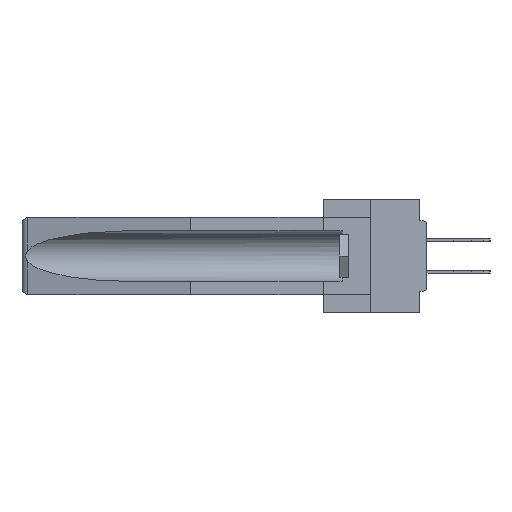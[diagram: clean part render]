
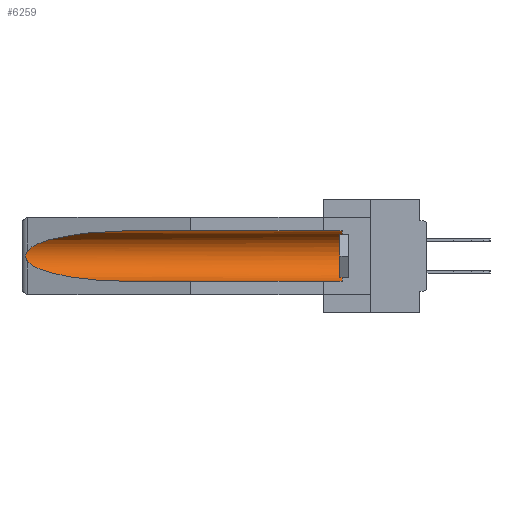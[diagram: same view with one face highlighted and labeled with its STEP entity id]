
A CAD part, left-side view. The second image highlights one B-rep face of the part: STEP entity #6259.
In plain terms, the highlighted cylindrical face has radius 2.857 mm (diameter 5.715 mm), a partial arc.
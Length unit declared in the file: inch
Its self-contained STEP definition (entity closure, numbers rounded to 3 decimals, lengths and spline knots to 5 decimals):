
#1116 = EDGE_CURVE ( 'NONE', #44423, #43679, #39667, .T. ) ;
#1277 = ORIENTED_EDGE ( 'NONE', *, *, #35236, .T. ) ;
#3763 = CARTESIAN_POINT ( 'NONE',  ( 0.21114, 1.30732, -0.059 ) ) ;
#4073 = DIRECTION ( 'NONE',  ( 0., 1., 0. ) ) ;
#4371 = CARTESIAN_POINT ( 'NONE',  ( 0.26537, 1.52718, -0.14972 ) ) ;
#4529 = CARTESIAN_POINT ( 'NONE',  ( 0.2675, 1.53308, -0.17534 ) ) ;
#5956 =( BOUNDED_CURVE ( )  B_SPLINE_CURVE ( 3, ( #27023, #19973, #22883, #26552 ),
 .UNSPECIFIED., .F., .F. ) 
 B_SPLINE_CURVE_WITH_KNOTS ( ( 4, 4 ),
 ( 0.1948, 1.5708 ),
 .UNSPECIFIED. ) 
 CURVE ( )  GEOMETRIC_REPRESENTATION_ITEM ( )  RATIONAL_B_SPLINE_CURVE ( ( 1., 0.848, 0.848, 1. ) ) 
 REPRESENTATION_ITEM ( '' )  );
#6259 = ADVANCED_FACE ( 'NONE', ( #20347 ), #40839, .F. ) ;
#7725 = DIRECTION ( 'NONE',  ( 0., -1., 0. ) ) ;
#7860 = CARTESIAN_POINT ( 'NONE',  ( 0.26654, 1.53092, -0.15636 ) ) ;
#7902 = CARTESIAN_POINT ( 'NONE',  ( 0.25451, 1.48313, -0.09465 ) ) ;
#8025 = CARTESIAN_POINT ( 'NONE',  ( 0.26655, 1.53094, -0.18657 ) ) ;
#8857 = EDGE_CURVE ( 'NONE', #40553, #43679, #5956, .T. ) ;
#9028 = LINE ( 'NONE', #21739, #17569 ) ;
#13466 = CARTESIAN_POINT ( 'NONE',  ( 0.155, -0.30754, -0.284 ) ) ;
#14746 = CARTESIAN_POINT ( 'NONE',  ( 0.155, 1.07973, -0.284 ) ) ;
#15071 = CARTESIAN_POINT ( 'NONE',  ( 0.2673, 1.53269, -0.17917 ) ) ;
#15427 = CARTESIAN_POINT ( 'NONE',  ( 0.26537, 1.52718, -0.14972 ) ) ;
#16601 = DIRECTION ( 'NONE',  ( 0., 1., 0. ) ) ;
#16863 = CARTESIAN_POINT ( 'NONE',  ( 0.155, 0.126, -0.059 ) ) ;
#17569 = VECTOR ( 'NONE', #4073, 39.37008 ) ;
#19849 = ORIENTED_EDGE ( 'NONE', *, *, #25614, .T. ) ;
#19970 = DIRECTION ( 'NONE',  ( 0., 0., 1. ) ) ;
#19973 = CARTESIAN_POINT ( 'NONE',  ( 0.25451, 1.48313, -0.24835 ) ) ;
#20347 = FACE_OUTER_BOUND ( 'NONE', #44023, .T. ) ;
#20691 = VERTEX_POINT ( 'NONE', #46167 ) ;
#21293 = AXIS2_PLACEMENT_3D ( 'NONE', #23169, #16601, #19970 ) ;
#21549 = CARTESIAN_POINT ( 'NONE',  ( 0.2673, 1.5327, -0.16383 ) ) ;
#21739 = CARTESIAN_POINT ( 'NONE',  ( 0.155, -0.30754, -0.059 ) ) ;
#22883 = CARTESIAN_POINT ( 'NONE',  ( 0.21114, 1.30732, -0.284 ) ) ;
#23169 = CARTESIAN_POINT ( 'NONE',  ( 0.155, -0.30754, -0.1715 ) ) ;
#25390 = EDGE_CURVE ( 'NONE', #43131, #20691, #31401, .T. ) ;
#25614 = EDGE_CURVE ( 'NONE', #44423, #38303, #40125, .T. ) ;
#26402 = CARTESIAN_POINT ( 'NONE',  ( 0.26597, 1.52961, -0.15275 ) ) ;
#26552 = CARTESIAN_POINT ( 'NONE',  ( 0.155, 1.07973, -0.284 ) ) ;
#27023 = CARTESIAN_POINT ( 'NONE',  ( 0.26537, 1.52718, -0.19328 ) ) ;
#27907 = AXIS2_PLACEMENT_3D ( 'NONE', #40448, #7725, #39821 ) ;
#27998 = EDGE_CURVE ( 'NONE', #20691, #40553, #39773, .T. ) ;
#29068 = ORIENTED_EDGE ( 'NONE', *, *, #27998, .T. ) ;
#29871 = CARTESIAN_POINT ( 'NONE',  ( 0.2675, 1.53308, -0.16763 ) ) ;
#31401 =( BOUNDED_CURVE ( )  B_SPLINE_CURVE ( 3, ( #43561, #3763, #7902, #15427 ),
 .UNSPECIFIED., .F., .F. ) 
 B_SPLINE_CURVE_WITH_KNOTS ( ( 4, 4 ),
 ( 4.71239, 6.08839 ),
 .UNSPECIFIED. ) 
 CURVE ( )  GEOMETRIC_REPRESENTATION_ITEM ( )  RATIONAL_B_SPLINE_CURVE ( ( 1., 0.848, 0.848, 1. ) ) 
 REPRESENTATION_ITEM ( '' )  );
#32290 = CARTESIAN_POINT ( 'NONE',  ( 0.26537, 1.52718, -0.19328 ) ) ;
#34081 = VECTOR ( 'NONE', #35104, 39.37008 ) ;
#35104 = DIRECTION ( 'NONE',  ( 0., 1., 0. ) ) ;
#35236 = EDGE_CURVE ( 'NONE', #38303, #43131, #9028, .T. ) ;
#37002 = CARTESIAN_POINT ( 'NONE',  ( 0.26597, 1.5296, -0.19026 ) ) ;
#37150 = CARTESIAN_POINT ( 'NONE',  ( 0.26537, 1.52718, -0.19328 ) ) ;
#38303 = VERTEX_POINT ( 'NONE', #16863 ) ;
#38572 = ORIENTED_EDGE ( 'NONE', *, *, #8857, .T. ) ;
#39029 = CARTESIAN_POINT ( 'NONE',  ( 0.155, 0.126, -0.284 ) ) ;
#39611 = CARTESIAN_POINT ( 'NONE',  ( 0.155, 1.07973, -0.059 ) ) ;
#39667 = LINE ( 'NONE', #13466, #34081 ) ;
#39773 = B_SPLINE_CURVE_WITH_KNOTS ( 'NONE', 3,
 ( #4371, #26402, #7860, #21549, #29871, #4529, #15071, #8025, #37002, #37150 ),
 .UNSPECIFIED., .F., .F.,
 ( 4, 2, 2, 2, 4 ),
 ( 0., 0.00029, 0.00058, 0.00087, 0.00117 ),
 .UNSPECIFIED. ) ;
#39821 = DIRECTION ( 'NONE',  ( 0., 0., 1. ) ) ;
#40125 = CIRCLE ( 'NONE', #27907, 0.1125 ) ;
#40448 = CARTESIAN_POINT ( 'NONE',  ( 0.155, 0.126, -0.1715 ) ) ;
#40553 = VERTEX_POINT ( 'NONE', #32290 ) ;
#40839 = CYLINDRICAL_SURFACE ( 'NONE', #21293, 0.1125 ) ;
#43131 = VERTEX_POINT ( 'NONE', #39611 ) ;
#43561 = CARTESIAN_POINT ( 'NONE',  ( 0.155, 1.07973, -0.059 ) ) ;
#43679 = VERTEX_POINT ( 'NONE', #14746 ) ;
#44023 = EDGE_LOOP ( 'NONE', ( #46688, #29068, #38572, #44156, #19849, #1277 ) ) ;
#44156 = ORIENTED_EDGE ( 'NONE', *, *, #1116, .F. ) ;
#44423 = VERTEX_POINT ( 'NONE', #39029 ) ;
#46167 = CARTESIAN_POINT ( 'NONE',  ( 0.26537, 1.52718, -0.14972 ) ) ;
#46688 = ORIENTED_EDGE ( 'NONE', *, *, #25390, .T. ) ;
